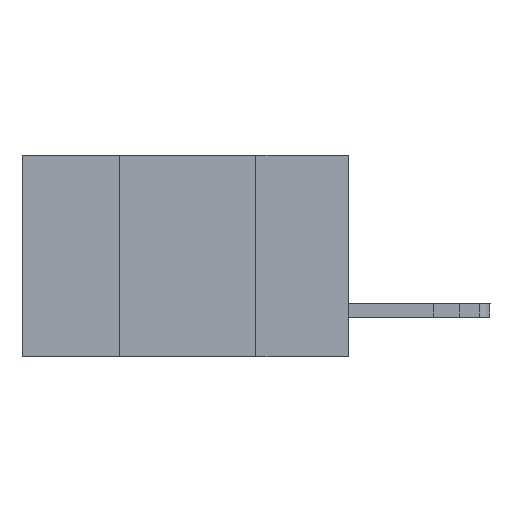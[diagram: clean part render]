
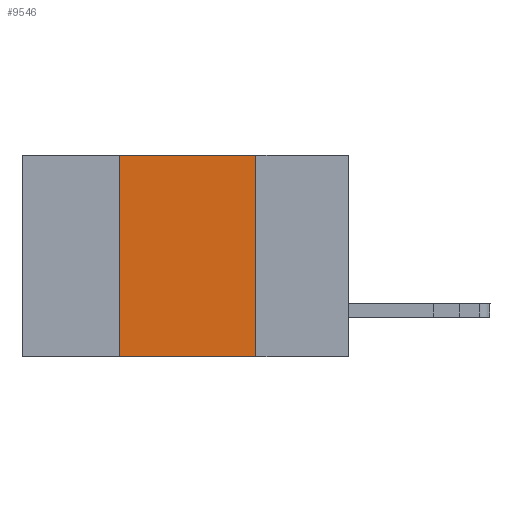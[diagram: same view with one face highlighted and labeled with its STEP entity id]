
A CAD part, left-side view. The second image highlights one B-rep face of the part: STEP entity #9546.
In plain terms, the highlighted planar face has unit normal (-1, 0, 0).
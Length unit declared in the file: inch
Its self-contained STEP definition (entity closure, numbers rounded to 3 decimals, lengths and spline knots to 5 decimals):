
#26 = CARTESIAN_POINT ( 'NONE',  ( 0., 0.17, 0. ) ) ;
#425 = VECTOR ( 'NONE', #3034, 39.37008 ) ;
#901 = DIRECTION ( 'NONE',  ( 1., 0., 0. ) ) ;
#1846 = PLANE ( 'NONE',  #3893 ) ;
#2039 = CARTESIAN_POINT ( 'NONE',  ( 0., 0.17, -0.37 ) ) ;
#2097 = CARTESIAN_POINT ( 'NONE',  ( 0., 0.17, -0.37 ) ) ;
#2365 = LINE ( 'NONE', #7971, #4687 ) ;
#2749 = LINE ( 'NONE', #2039, #425 ) ;
#2916 = EDGE_LOOP ( 'NONE', ( #5329, #5399, #5496, #5687 ) ) ;
#3034 = DIRECTION ( 'NONE',  ( 0., 0., -1. ) ) ;
#3076 = DIRECTION ( 'NONE',  ( 0., -1., 0. ) ) ;
#3149 = LINE ( 'NONE', #9015, #11355 ) ;
#3589 = VERTEX_POINT ( 'NONE', #3990 ) ;
#3722 = VERTEX_POINT ( 'NONE', #26 ) ;
#3893 = AXIS2_PLACEMENT_3D ( 'NONE', #11722, #901, #7790 ) ;
#3990 = CARTESIAN_POINT ( 'NONE',  ( 0., 0.42, 0. ) ) ;
#4625 = VECTOR ( 'NONE', #7785, 39.37008 ) ;
#4687 = VECTOR ( 'NONE', #8996, 39.37008 ) ;
#4890 = VERTEX_POINT ( 'NONE', #2097 ) ;
#5329 = ORIENTED_EDGE ( 'NONE', *, *, #8310, .F. ) ;
#5399 = ORIENTED_EDGE ( 'NONE', *, *, #10361, .F. ) ;
#5496 = ORIENTED_EDGE ( 'NONE', *, *, #11000, .F. ) ;
#5687 = ORIENTED_EDGE ( 'NONE', *, *, #7636, .T. ) ;
#7523 = LINE ( 'NONE', #12642, #4625 ) ;
#7636 = EDGE_CURVE ( 'NONE', #10445, #4890, #7523, .T. ) ;
#7785 = DIRECTION ( 'NONE',  ( 0., -1., 0. ) ) ;
#7790 = DIRECTION ( 'NONE',  ( 0., 0., -1. ) ) ;
#7971 = CARTESIAN_POINT ( 'NONE',  ( 0., 0.42, -0.37 ) ) ;
#8117 = CARTESIAN_POINT ( 'NONE',  ( 0., 0.42, -0.37 ) ) ;
#8310 = EDGE_CURVE ( 'NONE', #3722, #4890, #2749, .T. ) ;
#8996 = DIRECTION ( 'NONE',  ( 0., 0., 1. ) ) ;
#9015 = CARTESIAN_POINT ( 'NONE',  ( 0., 0.6, 0. ) ) ;
#9546 = ADVANCED_FACE ( 'NONE', ( #9867 ), #1846, .F. ) ;
#9867 = FACE_OUTER_BOUND ( 'NONE', #2916, .T. ) ;
#10361 = EDGE_CURVE ( 'NONE', #3589, #3722, #3149, .T. ) ;
#10445 = VERTEX_POINT ( 'NONE', #8117 ) ;
#11000 = EDGE_CURVE ( 'NONE', #10445, #3589, #2365, .T. ) ;
#11355 = VECTOR ( 'NONE', #3076, 39.37008 ) ;
#11722 = CARTESIAN_POINT ( 'NONE',  ( 0., 0.6, 0. ) ) ;
#12642 = CARTESIAN_POINT ( 'NONE',  ( 0., 0.6, -0.37 ) ) ;
